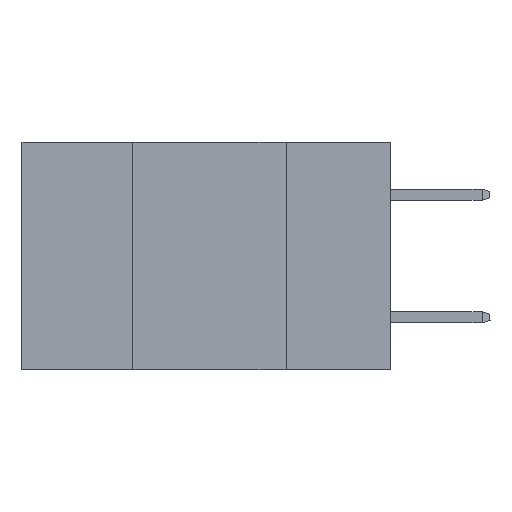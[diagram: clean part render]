
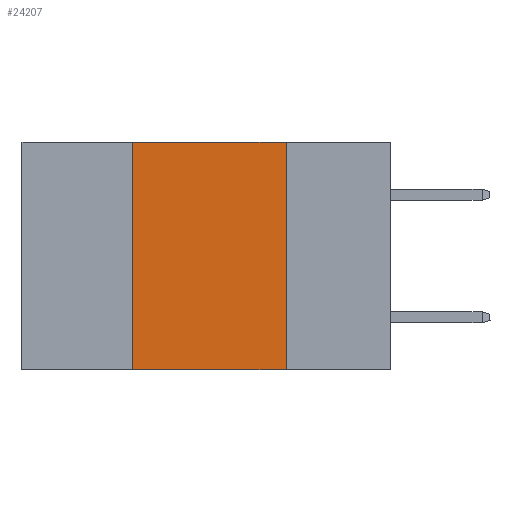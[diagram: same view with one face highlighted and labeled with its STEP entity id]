
A CAD part, left-side view. The second image highlights one B-rep face of the part: STEP entity #24207.
In plain terms, the highlighted planar face has unit normal (-1, 0, 0).
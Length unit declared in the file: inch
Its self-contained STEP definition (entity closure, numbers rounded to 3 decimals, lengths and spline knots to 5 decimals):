
#224 = ORIENTED_EDGE ( 'NONE', *, *, #12585, .F. ) ;
#475 = VERTEX_POINT ( 'NONE', #21736 ) ;
#969 = DIRECTION ( 'NONE',  ( 0., 0., -1. ) ) ;
#1213 = PLANE ( 'NONE',  #3523 ) ;
#1340 = CARTESIAN_POINT ( 'NONE',  ( 0., 0.42, 0. ) ) ;
#2169 = EDGE_CURVE ( 'NONE', #475, #19480, #9277, .T. ) ;
#3081 = EDGE_LOOP ( 'NONE', ( #23192, #9465, #224, #11081 ) ) ;
#3523 = AXIS2_PLACEMENT_3D ( 'NONE', #4704, #12513, #969 ) ;
#4704 = CARTESIAN_POINT ( 'NONE',  ( 0., 0.6, 0. ) ) ;
#4763 = VERTEX_POINT ( 'NONE', #22188 ) ;
#4903 = EDGE_CURVE ( 'NONE', #4763, #19480, #13518, .T. ) ;
#5316 = LINE ( 'NONE', #1340, #18343 ) ;
#6101 = VECTOR ( 'NONE', #18528, 39.37008 ) ;
#6582 = FACE_OUTER_BOUND ( 'NONE', #3081, .T. ) ;
#8092 = CARTESIAN_POINT ( 'NONE',  ( 0., 0.42, 0. ) ) ;
#8772 = VERTEX_POINT ( 'NONE', #8092 ) ;
#9277 = LINE ( 'NONE', #13242, #6101 ) ;
#9465 = ORIENTED_EDGE ( 'NONE', *, *, #15534, .F. ) ;
#10176 = DIRECTION ( 'NONE',  ( 0., -1., 0. ) ) ;
#11081 = ORIENTED_EDGE ( 'NONE', *, *, #2169, .T. ) ;
#11668 = CARTESIAN_POINT ( 'NONE',  ( 0., 0.6, 0. ) ) ;
#12513 = DIRECTION ( 'NONE',  ( 1., 0., 0. ) ) ;
#12585 = EDGE_CURVE ( 'NONE', #475, #8772, #5316, .T. ) ;
#13242 = CARTESIAN_POINT ( 'NONE',  ( 0., 0.6, -0.37 ) ) ;
#13518 = LINE ( 'NONE', #17215, #20904 ) ;
#14079 = VECTOR ( 'NONE', #10176, 39.37008 ) ;
#15534 = EDGE_CURVE ( 'NONE', #8772, #4763, #15743, .T. ) ;
#15743 = LINE ( 'NONE', #11668, #14079 ) ;
#17215 = CARTESIAN_POINT ( 'NONE',  ( 0., 0.17, 0. ) ) ;
#18008 = CARTESIAN_POINT ( 'NONE',  ( 0., 0.17, -0.37 ) ) ;
#18343 = VECTOR ( 'NONE', #22147, 39.37008 ) ;
#18528 = DIRECTION ( 'NONE',  ( 0., -1., 0. ) ) ;
#19480 = VERTEX_POINT ( 'NONE', #18008 ) ;
#20904 = VECTOR ( 'NONE', #21056, 39.37008 ) ;
#21056 = DIRECTION ( 'NONE',  ( 0., 0., -1. ) ) ;
#21736 = CARTESIAN_POINT ( 'NONE',  ( 0., 0.42, -0.37 ) ) ;
#22147 = DIRECTION ( 'NONE',  ( 0., 0., 1. ) ) ;
#22188 = CARTESIAN_POINT ( 'NONE',  ( 0., 0.17, 0. ) ) ;
#23192 = ORIENTED_EDGE ( 'NONE', *, *, #4903, .F. ) ;
#24207 = ADVANCED_FACE ( 'NONE', ( #6582 ), #1213, .F. ) ;
